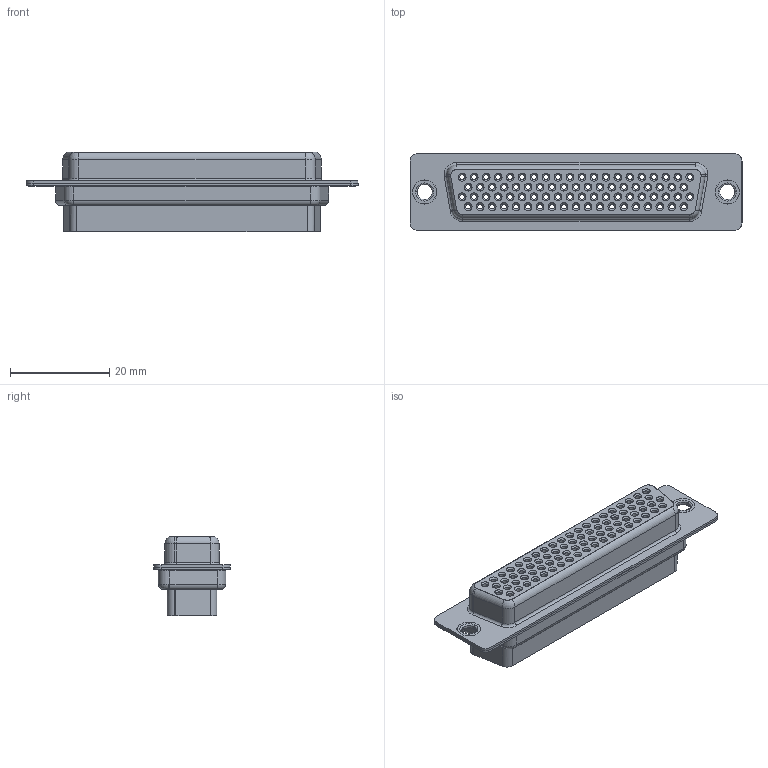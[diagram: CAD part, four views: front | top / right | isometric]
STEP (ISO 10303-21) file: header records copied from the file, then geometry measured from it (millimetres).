
FILE_DESCRIPTION (( 'STEP AP203' ), '1' );
FILE_NAME ('638-078-010-241.STEP', '2020-07-18T16:53:16', ( '' ), ( '' ), 'SwSTEP 2.0', 'SolidWorks 2020', '' );
FILE_SCHEMA (( 'CONFIG_CONTROL_DESIGN' ));
Length unit declared in the file: millimetre
Products named in the file (5): 638 Thru Hole Rivet; 638-078-010-241; 638 Shell Rear_78 Contacts; 638 Shell Front_78 Contacts; 638 Housing_78 Contacts HP
Assembly tree (5 placements, depth 2):
  638-078-010-241
    638 Housing_78 Contacts HP
    638 Shell Front_78 Contacts
    638 Shell Rear_78 Contacts
    638 Thru Hole Rivet  x2
Bounding box: 67 x 15.4 x 16.1 mm (x, y, z)
Volume: 6335.1 mm3; surface area: 14566.6 mm2
Topology: 5 solids, 5 shells, 1267 faces, 2787 edges, 1775 vertices
Faces by surface type: cylinder 745, plane 301, cone 156, torus 65
Entity records: 35888 total; most frequent: DIRECTION 6899, CARTESIAN_POINT 5936, ORIENTED_EDGE 5494, AXIS2_PLACEMENT_3D 2942, EDGE_CURVE 2747, VERTEX_POINT 1751, CIRCLE 1687, EDGE_LOOP 1660
